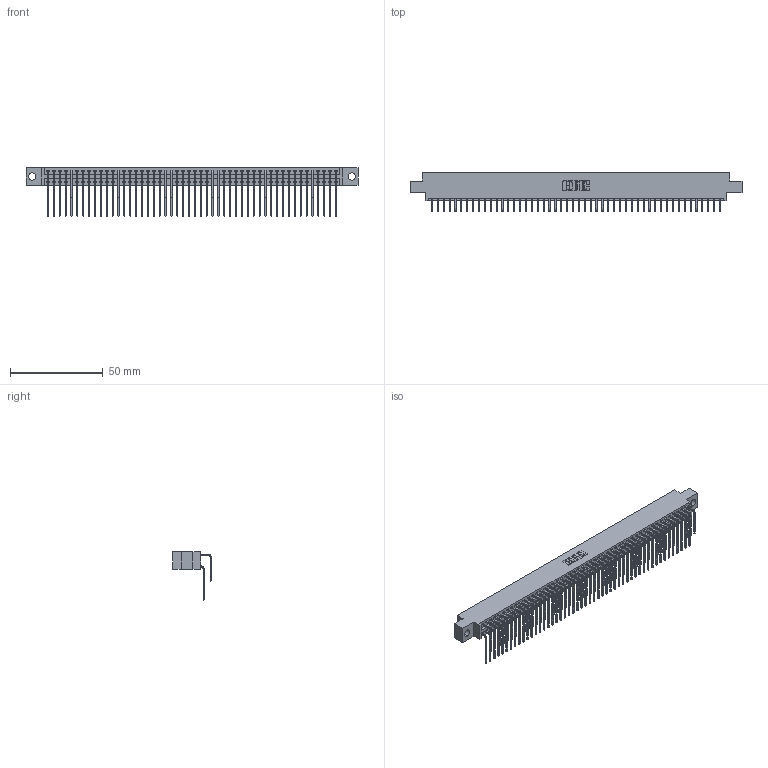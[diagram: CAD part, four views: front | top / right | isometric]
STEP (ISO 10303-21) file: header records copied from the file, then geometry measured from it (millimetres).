
FILE_DESCRIPTION (( 'STEP AP203' ), '1' );
FILE_NAME ('346-100-559-804.STEP', '2018-08-30T11:45:12', ( '' ), ( '' ), 'SwSTEP 2.0', 'SolidWorks 2016', '' );
FILE_SCHEMA (( 'CONFIG_CONTROL_DESIGN' ));
Length unit declared in the file: inch
Products named in the file (4): 346-100-559-804; 346 Part_0.170 Offset - 0.156 Dia-TH; 345-292-001_558 559 Tail - 1; 345-292-001_559 Tail - 2
Assembly tree (101 placements, depth 2):
  346-100-559-804
    346 Part_0.170 Offset - 0.156 Dia-TH
    345-292-001_558 559 Tail - 1  x50
    345-292-001_559 Tail - 2  x50
Bounding box: 179.32 x 20.89 x 26.16 mm (x, y, z)
Volume: 17882.9 mm3; surface area: 27467.4 mm2
Topology: 101 solids, 101 shells, 5526 faces, 16441 edges, 10826 vertices
Faces by surface type: plane 3780, cylinder 1746
Entity records: 33473 total; most frequent: CARTESIAN_POINT 5559, ORIENTED_EDGE 5442, DIRECTION 4921, EDGE_CURVE 2721, LINE 2349, VECTOR 2349, VERTEX_POINT 1810, AXIS2_PLACEMENT_3D 1286
